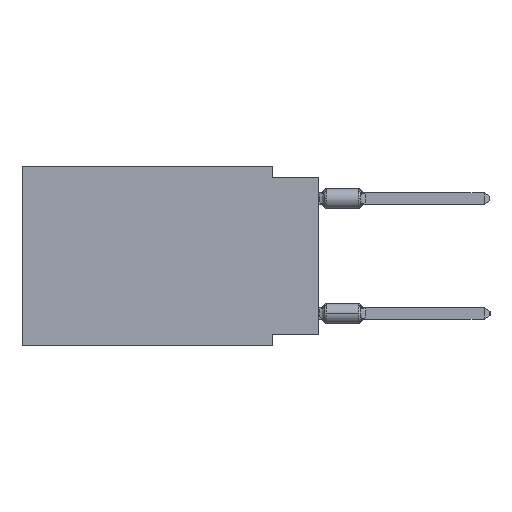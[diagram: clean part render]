
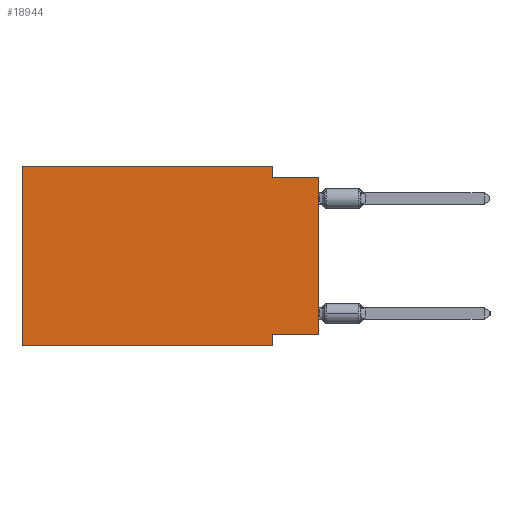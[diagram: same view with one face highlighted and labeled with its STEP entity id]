
A CAD part, left-side view. The second image highlights one B-rep face of the part: STEP entity #18944.
In plain terms, the highlighted planar face has unit normal (-1, 0, 0).
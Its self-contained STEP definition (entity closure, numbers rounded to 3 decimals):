
#589 = CARTESIAN_POINT ( 'NONE',  ( 0., 0., -9.271 ) ) ;
#764 = ORIENTED_EDGE ( 'NONE', *, *, #37405, .F. ) ;
#2378 = VECTOR ( 'NONE', #49717, 1000. ) ;
#4272 = VERTEX_POINT ( 'NONE', #8279 ) ;
#4451 = LINE ( 'NONE', #12400, #25874 ) ;
#8279 = CARTESIAN_POINT ( 'NONE',  ( 0., 2.54, -0.635 ) ) ;
#8654 = VECTOR ( 'NONE', #33742, 1000. ) ;
#9467 = CARTESIAN_POINT ( 'NONE',  ( 0., 16.383, 0. ) ) ;
#9976 = PLANE ( 'NONE',  #48168 ) ;
#10095 = CARTESIAN_POINT ( 'NONE',  ( 0., 16.383, 0. ) ) ;
#11193 = LINE ( 'NONE', #30763, #27117 ) ;
#11323 = LINE ( 'NONE', #42968, #11478 ) ;
#11478 = VECTOR ( 'NONE', #38601, 1000. ) ;
#12070 = LINE ( 'NONE', #20293, #39692 ) ;
#12400 = CARTESIAN_POINT ( 'NONE',  ( 0., 2.54, 0. ) ) ;
#13646 = ORIENTED_EDGE ( 'NONE', *, *, #19935, .F. ) ;
#13821 = DIRECTION ( 'NONE',  ( 0., 0., -1. ) ) ;
#15691 = DIRECTION ( 'NONE',  ( 0., -1., 0. ) ) ;
#18042 = CARTESIAN_POINT ( 'NONE',  ( 0., 0., 0. ) ) ;
#18944 = ADVANCED_FACE ( 'NONE', ( #49324 ), #9976, .F. ) ;
#19140 = VERTEX_POINT ( 'NONE', #47251 ) ;
#19935 = EDGE_CURVE ( 'NONE', #21415, #33633, #11323, .T. ) ;
#20293 = CARTESIAN_POINT ( 'NONE',  ( 0., 0., -0.635 ) ) ;
#20471 = EDGE_LOOP ( 'NONE', ( #47141, #48239, #764, #32771, #44892, #36792, #13646, #41714 ) ) ;
#21305 = CARTESIAN_POINT ( 'NONE',  ( 0., 2.54, -9.271 ) ) ;
#21415 = VERTEX_POINT ( 'NONE', #21305 ) ;
#22296 = EDGE_CURVE ( 'NONE', #37346, #21415, #11193, .T. ) ;
#23643 = CARTESIAN_POINT ( 'NONE',  ( 0., 16.383, 0. ) ) ;
#24112 = VECTOR ( 'NONE', #41477, 1000. ) ;
#25501 = VECTOR ( 'NONE', #39345, 1000. ) ;
#25874 = VECTOR ( 'NONE', #40166, 1000. ) ;
#26914 = EDGE_CURVE ( 'NONE', #19140, #33633, #37898, .T. ) ;
#27117 = VECTOR ( 'NONE', #38721, 1000. ) ;
#28000 = CARTESIAN_POINT ( 'NONE',  ( 0., 16.383, 0. ) ) ;
#29648 = VERTEX_POINT ( 'NONE', #29896 ) ;
#29896 = CARTESIAN_POINT ( 'NONE',  ( 0., 2.54, 0. ) ) ;
#29897 = LINE ( 'NONE', #18042, #8654 ) ;
#30611 = VERTEX_POINT ( 'NONE', #28000 ) ;
#30763 = CARTESIAN_POINT ( 'NONE',  ( 0., 0., -9.271 ) ) ;
#31892 = LINE ( 'NONE', #23643, #25501 ) ;
#32771 = ORIENTED_EDGE ( 'NONE', *, *, #49612, .F. ) ;
#33513 = EDGE_CURVE ( 'NONE', #4272, #50602, #12070, .T. ) ;
#33633 = VERTEX_POINT ( 'NONE', #40095 ) ;
#33742 = DIRECTION ( 'NONE',  ( 0., 0., 1. ) ) ;
#34046 = CARTESIAN_POINT ( 'NONE',  ( 0., 16.383, -9.906 ) ) ;
#34102 = EDGE_CURVE ( 'NONE', #19140, #30611, #41990, .T. ) ;
#36792 = ORIENTED_EDGE ( 'NONE', *, *, #26914, .T. ) ;
#37346 = VERTEX_POINT ( 'NONE', #589 ) ;
#37405 = EDGE_CURVE ( 'NONE', #29648, #4272, #4451, .T. ) ;
#37898 = LINE ( 'NONE', #34046, #2378 ) ;
#38258 = CARTESIAN_POINT ( 'NONE',  ( 0., 0., -0.635 ) ) ;
#38404 = EDGE_CURVE ( 'NONE', #37346, #50602, #29897, .T. ) ;
#38601 = DIRECTION ( 'NONE',  ( 0., 0., -1. ) ) ;
#38721 = DIRECTION ( 'NONE',  ( 0., 1., 0. ) ) ;
#39345 = DIRECTION ( 'NONE',  ( 0., -1., 0. ) ) ;
#39692 = VECTOR ( 'NONE', #15691, 1000. ) ;
#40095 = CARTESIAN_POINT ( 'NONE',  ( 0., 2.54, -9.906 ) ) ;
#40166 = DIRECTION ( 'NONE',  ( 0., 0., -1. ) ) ;
#40843 = DIRECTION ( 'NONE',  ( 1., 0., 0. ) ) ;
#41477 = DIRECTION ( 'NONE',  ( 0., 0., 1. ) ) ;
#41714 = ORIENTED_EDGE ( 'NONE', *, *, #22296, .F. ) ;
#41990 = LINE ( 'NONE', #10095, #24112 ) ;
#42968 = CARTESIAN_POINT ( 'NONE',  ( 0., 2.54, -9.906 ) ) ;
#44892 = ORIENTED_EDGE ( 'NONE', *, *, #34102, .F. ) ;
#47141 = ORIENTED_EDGE ( 'NONE', *, *, #38404, .T. ) ;
#47251 = CARTESIAN_POINT ( 'NONE',  ( 0., 16.383, -9.906 ) ) ;
#48168 = AXIS2_PLACEMENT_3D ( 'NONE', #9467, #40843, #13821 ) ;
#48239 = ORIENTED_EDGE ( 'NONE', *, *, #33513, .F. ) ;
#49324 = FACE_OUTER_BOUND ( 'NONE', #20471, .T. ) ;
#49612 = EDGE_CURVE ( 'NONE', #30611, #29648, #31892, .T. ) ;
#49717 = DIRECTION ( 'NONE',  ( 0., -1., 0. ) ) ;
#50602 = VERTEX_POINT ( 'NONE', #38258 ) ;
